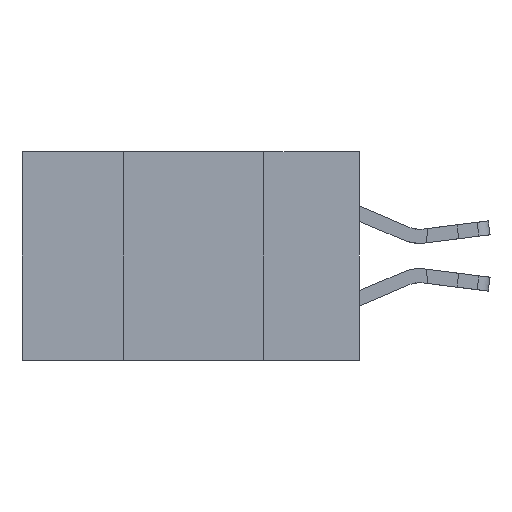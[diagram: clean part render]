
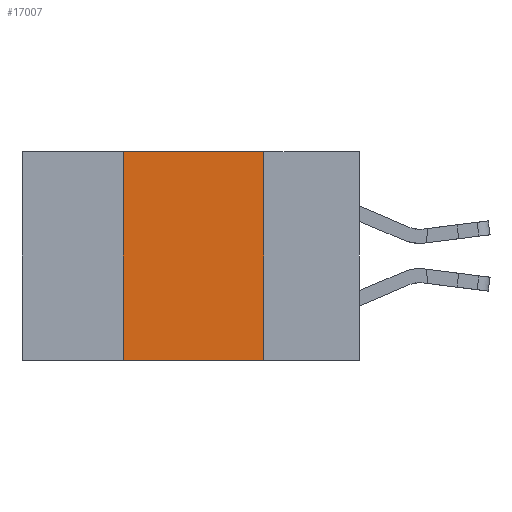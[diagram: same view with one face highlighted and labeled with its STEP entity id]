
A CAD part, left-side view. The second image highlights one B-rep face of the part: STEP entity #17007.
In plain terms, the highlighted planar face has unit normal (-1, 0, 0).
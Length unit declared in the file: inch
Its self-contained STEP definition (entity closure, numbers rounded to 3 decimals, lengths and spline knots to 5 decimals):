
#2634 = AXIS2_PLACEMENT_3D ( 'NONE', #11192, #27292, #13858 ) ;
#3357 = CARTESIAN_POINT ( 'NONE',  ( 0., 0.17, 0. ) ) ;
#3361 = VERTEX_POINT ( 'NONE', #22256 ) ;
#3543 = LINE ( 'NONE', #14463, #18164 ) ;
#4196 = EDGE_CURVE ( 'NONE', #7068, #3361, #3543, .T. ) ;
#4969 = CARTESIAN_POINT ( 'NONE',  ( 0., 0.42, 0. ) ) ;
#5857 = ORIENTED_EDGE ( 'NONE', *, *, #17534, .F. ) ;
#6416 = ORIENTED_EDGE ( 'NONE', *, *, #23850, .F. ) ;
#7068 = VERTEX_POINT ( 'NONE', #10399 ) ;
#7360 = VERTEX_POINT ( 'NONE', #17891 ) ;
#8386 = VECTOR ( 'NONE', #10522, 39.37008 ) ;
#8864 = DIRECTION ( 'NONE',  ( 0., 0., -1. ) ) ;
#10399 = CARTESIAN_POINT ( 'NONE',  ( 0., 0.42, -0.37 ) ) ;
#10522 = DIRECTION ( 'NONE',  ( 0., -1., 0. ) ) ;
#11192 = CARTESIAN_POINT ( 'NONE',  ( 0., 0.6, 0. ) ) ;
#12708 = LINE ( 'NONE', #4969, #26185 ) ;
#13070 = CARTESIAN_POINT ( 'NONE',  ( 0., 0.6, 0. ) ) ;
#13858 = DIRECTION ( 'NONE',  ( 0., 0., -1. ) ) ;
#14463 = CARTESIAN_POINT ( 'NONE',  ( 0., 0.6, -0.37 ) ) ;
#14826 = FACE_OUTER_BOUND ( 'NONE', #29509, .T. ) ;
#15211 = ORIENTED_EDGE ( 'NONE', *, *, #33965, .F. ) ;
#17007 = ADVANCED_FACE ( 'NONE', ( #14826 ), #21901, .F. ) ;
#17534 = EDGE_CURVE ( 'NONE', #7068, #23346, #12708, .T. ) ;
#17719 = ORIENTED_EDGE ( 'NONE', *, *, #4196, .T. ) ;
#17891 = CARTESIAN_POINT ( 'NONE',  ( 0., 0.17, 0. ) ) ;
#18164 = VECTOR ( 'NONE', #33810, 39.37008 ) ;
#18314 = LINE ( 'NONE', #3357, #25456 ) ;
#21901 = PLANE ( 'NONE',  #2634 ) ;
#22256 = CARTESIAN_POINT ( 'NONE',  ( 0., 0.17, -0.37 ) ) ;
#22642 = LINE ( 'NONE', #13070, #8386 ) ;
#23346 = VERTEX_POINT ( 'NONE', #33865 ) ;
#23850 = EDGE_CURVE ( 'NONE', #7360, #3361, #18314, .T. ) ;
#25456 = VECTOR ( 'NONE', #8864, 39.37008 ) ;
#25957 = DIRECTION ( 'NONE',  ( 0., 0., 1. ) ) ;
#26185 = VECTOR ( 'NONE', #25957, 39.37008 ) ;
#27292 = DIRECTION ( 'NONE',  ( 1., 0., 0. ) ) ;
#29509 = EDGE_LOOP ( 'NONE', ( #6416, #15211, #5857, #17719 ) ) ;
#33810 = DIRECTION ( 'NONE',  ( 0., -1., 0. ) ) ;
#33865 = CARTESIAN_POINT ( 'NONE',  ( 0., 0.42, 0. ) ) ;
#33965 = EDGE_CURVE ( 'NONE', #23346, #7360, #22642, .T. ) ;
